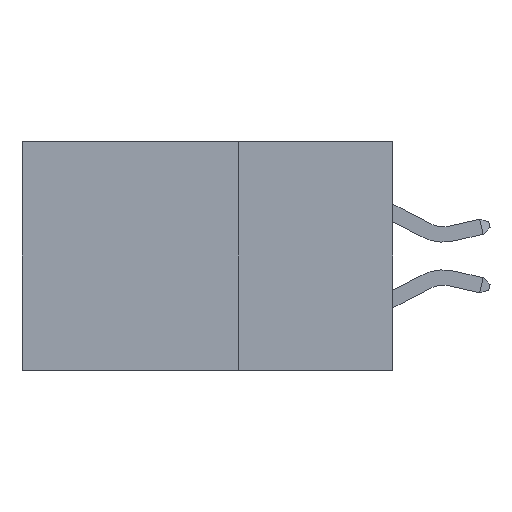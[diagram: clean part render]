
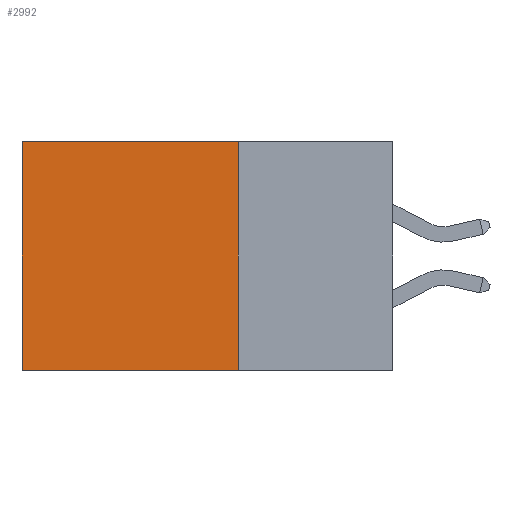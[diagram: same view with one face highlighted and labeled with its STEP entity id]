
A CAD part, left-side view. The second image highlights one B-rep face of the part: STEP entity #2992.
In plain terms, the highlighted planar face has unit normal (-1, 0, 0).
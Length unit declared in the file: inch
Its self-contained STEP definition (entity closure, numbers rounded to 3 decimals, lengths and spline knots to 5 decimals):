
#138 = DIRECTION ( 'NONE',  ( 0., 1., 0. ) ) ;
#278 = ORIENTED_EDGE ( 'NONE', *, *, #558, .T. ) ;
#558 = EDGE_CURVE ( 'NONE', #12313, #7799, #4335, .T. ) ;
#598 = CARTESIAN_POINT ( 'NONE',  ( 0.2875, 0.6, 0. ) ) ;
#867 = DIRECTION ( 'NONE',  ( 0., 0., -1. ) ) ;
#1116 = EDGE_LOOP ( 'NONE', ( #11593, #13734, #1402, #278 ) ) ;
#1402 = ORIENTED_EDGE ( 'NONE', *, *, #16140, .F. ) ;
#1509 = CARTESIAN_POINT ( 'NONE',  ( 0.2875, 0.25, 0. ) ) ;
#1567 = CARTESIAN_POINT ( 'NONE',  ( 0.2875, 0.25, 0. ) ) ;
#2992 = ADVANCED_FACE ( 'NONE', ( #16793 ), #9186, .F. ) ;
#3708 = DIRECTION ( 'NONE',  ( 0., 0., -1. ) ) ;
#4106 = DIRECTION ( 'NONE',  ( 0., 1., 0. ) ) ;
#4235 = VERTEX_POINT ( 'NONE', #6226 ) ;
#4335 = LINE ( 'NONE', #1509, #9418 ) ;
#4592 = LINE ( 'NONE', #12553, #12958 ) ;
#4928 = VERTEX_POINT ( 'NONE', #7749 ) ;
#6091 = LINE ( 'NONE', #17867, #11160 ) ;
#6226 = CARTESIAN_POINT ( 'NONE',  ( 0.2875, 0.6, -0.37 ) ) ;
#6938 = LINE ( 'NONE', #598, #11140 ) ;
#7749 = CARTESIAN_POINT ( 'NONE',  ( 0.2875, 0.25, -0.37 ) ) ;
#7799 = VERTEX_POINT ( 'NONE', #15799 ) ;
#9186 = PLANE ( 'NONE',  #17449 ) ;
#9245 = CARTESIAN_POINT ( 'NONE',  ( 0.2875, 0.25, 0. ) ) ;
#9418 = VECTOR ( 'NONE', #138, 39.37008 ) ;
#9429 = DIRECTION ( 'NONE',  ( 0., 0., -1. ) ) ;
#11140 = VECTOR ( 'NONE', #867, 39.37008 ) ;
#11160 = VECTOR ( 'NONE', #9429, 39.37008 ) ;
#11593 = ORIENTED_EDGE ( 'NONE', *, *, #16600, .T. ) ;
#12313 = VERTEX_POINT ( 'NONE', #1567 ) ;
#12553 = CARTESIAN_POINT ( 'NONE',  ( 0.2875, 0.25, -0.37 ) ) ;
#12958 = VECTOR ( 'NONE', #4106, 39.37008 ) ;
#13734 = ORIENTED_EDGE ( 'NONE', *, *, #17405, .F. ) ;
#15799 = CARTESIAN_POINT ( 'NONE',  ( 0.2875, 0.6, 0. ) ) ;
#16140 = EDGE_CURVE ( 'NONE', #12313, #4928, #6091, .T. ) ;
#16243 = DIRECTION ( 'NONE',  ( 1., 0., 0. ) ) ;
#16600 = EDGE_CURVE ( 'NONE', #7799, #4235, #6938, .T. ) ;
#16793 = FACE_OUTER_BOUND ( 'NONE', #1116, .T. ) ;
#17405 = EDGE_CURVE ( 'NONE', #4928, #4235, #4592, .T. ) ;
#17449 = AXIS2_PLACEMENT_3D ( 'NONE', #9245, #16243, #3708 ) ;
#17867 = CARTESIAN_POINT ( 'NONE',  ( 0.2875, 0.25, 0. ) ) ;
